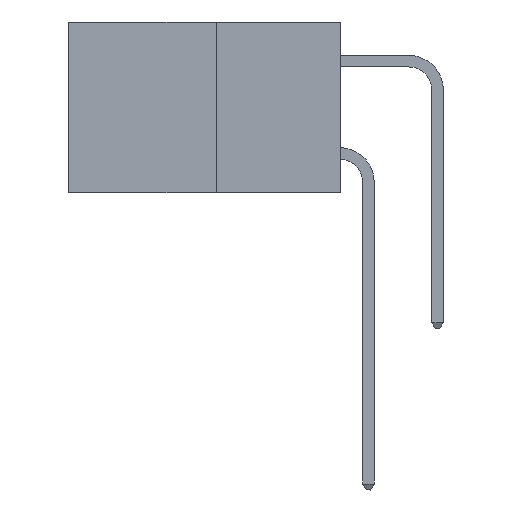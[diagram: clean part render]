
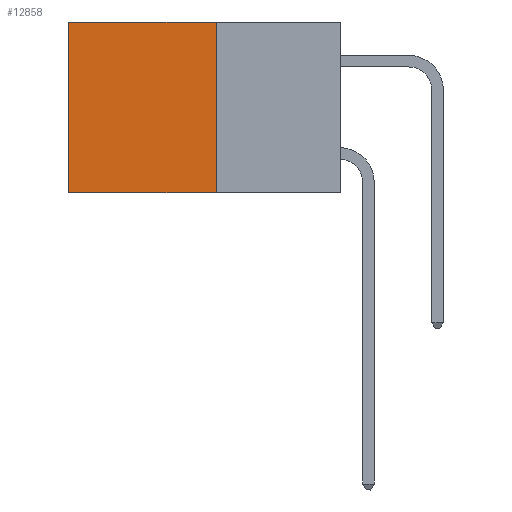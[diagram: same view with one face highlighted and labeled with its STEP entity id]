
A CAD part, left-side view. The second image highlights one B-rep face of the part: STEP entity #12858.
In plain terms, the highlighted planar face has unit normal (-1, 0, 0).
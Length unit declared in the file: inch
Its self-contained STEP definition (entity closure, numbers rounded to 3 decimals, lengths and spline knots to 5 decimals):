
#153 = ORIENTED_EDGE ( 'NONE', *, *, #1961, .F. ) ;
#318 = EDGE_CURVE ( 'NONE', #6145, #7419, #12407, .T. ) ;
#1647 = LINE ( 'NONE', #4335, #4588 ) ;
#1961 = EDGE_CURVE ( 'NONE', #7419, #4859, #1647, .T. ) ;
#2660 = CARTESIAN_POINT ( 'NONE',  ( 0.277, 0.27, 0. ) ) ;
#3778 = EDGE_CURVE ( 'NONE', #9022, #4859, #9755, .T. ) ;
#4335 = CARTESIAN_POINT ( 'NONE',  ( 0.277, 0.27, -0.37 ) ) ;
#4588 = VECTOR ( 'NONE', #6642, 39.37008 ) ;
#4859 = VERTEX_POINT ( 'NONE', #12718 ) ;
#5325 = EDGE_LOOP ( 'NONE', ( #13765, #153, #11475, #11083 ) ) ;
#5835 = VECTOR ( 'NONE', #9380, 39.37008 ) ;
#6145 = VERTEX_POINT ( 'NONE', #2660 ) ;
#6586 = AXIS2_PLACEMENT_3D ( 'NONE', #12797, #14026, #6671 ) ;
#6642 = DIRECTION ( 'NONE',  ( 0., 1., 0. ) ) ;
#6671 = DIRECTION ( 'NONE',  ( 0., 0., -1. ) ) ;
#7419 = VERTEX_POINT ( 'NONE', #15934 ) ;
#8284 = LINE ( 'NONE', #11167, #14400 ) ;
#8608 = CARTESIAN_POINT ( 'NONE',  ( 0.277, 0.27, -0.37 ) ) ;
#9022 = VERTEX_POINT ( 'NONE', #10578 ) ;
#9380 = DIRECTION ( 'NONE',  ( 0., 0., -1. ) ) ;
#9639 = DIRECTION ( 'NONE',  ( 0., 1., 0. ) ) ;
#9755 = LINE ( 'NONE', #11693, #12609 ) ;
#10337 = FACE_OUTER_BOUND ( 'NONE', #5325, .T. ) ;
#10578 = CARTESIAN_POINT ( 'NONE',  ( 0.277, 0.59, 0. ) ) ;
#10702 = EDGE_CURVE ( 'NONE', #6145, #9022, #8284, .T. ) ;
#11083 = ORIENTED_EDGE ( 'NONE', *, *, #10702, .T. ) ;
#11167 = CARTESIAN_POINT ( 'NONE',  ( 0.277, 0.27, 0. ) ) ;
#11475 = ORIENTED_EDGE ( 'NONE', *, *, #318, .F. ) ;
#11569 = PLANE ( 'NONE',  #6586 ) ;
#11693 = CARTESIAN_POINT ( 'NONE',  ( 0.277, 0.59, -0.37 ) ) ;
#11812 = DIRECTION ( 'NONE',  ( 0., 0., -1. ) ) ;
#12407 = LINE ( 'NONE', #8608, #5835 ) ;
#12609 = VECTOR ( 'NONE', #11812, 39.37008 ) ;
#12718 = CARTESIAN_POINT ( 'NONE',  ( 0.277, 0.59, -0.37 ) ) ;
#12797 = CARTESIAN_POINT ( 'NONE',  ( 0.277, 0.27, -0.37 ) ) ;
#12858 = ADVANCED_FACE ( 'NONE', ( #10337 ), #11569, .F. ) ;
#13765 = ORIENTED_EDGE ( 'NONE', *, *, #3778, .T. ) ;
#14026 = DIRECTION ( 'NONE',  ( 1., 0., 0. ) ) ;
#14400 = VECTOR ( 'NONE', #9639, 39.37008 ) ;
#15934 = CARTESIAN_POINT ( 'NONE',  ( 0.277, 0.27, -0.37 ) ) ;
